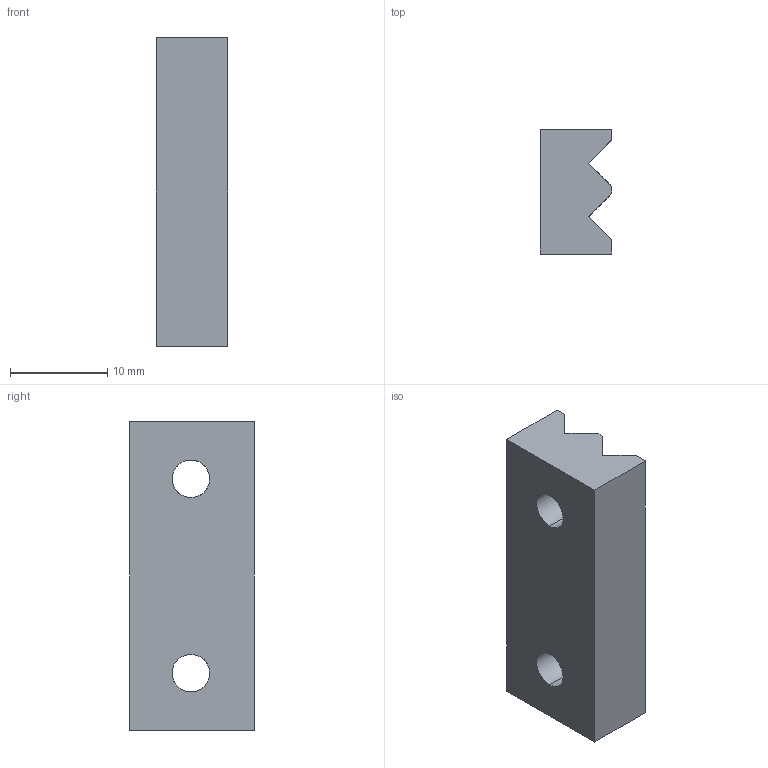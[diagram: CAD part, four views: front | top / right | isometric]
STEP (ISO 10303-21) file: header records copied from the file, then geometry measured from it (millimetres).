
FILE_DESCRIPTION (( 'STEP AP214' ), '1' );
FILE_NAME ('ForeGrip-Retainer.STEP', '2015-01-24T03:30:35', ( 'WarFairy' ), ( '' ), 'SwSTEP 2.0', 'SolidWorks 2013', '' );
FILE_SCHEMA (( 'AUTOMOTIVE_DESIGN' ));
Length unit declared in the file: inch
Products named in the file (1): ForeGrip-Retainer
Bounding box: 7.4 x 12.83 x 31.75 mm (x, y, z)
Volume: 2488.5 mm3; surface area: 1681.1 mm2
Topology: 1 solids, 1 shells, 18 faces, 54 edges, 36 vertices
Faces by surface type: plane 14, cylinder 4
Entity records: 710 total; most frequent: CARTESIAN_POINT 121, ORIENTED_EDGE 108, DIRECTION 100, EDGE_CURVE 54, VECTOR 38, LINE 38, VERTEX_POINT 36, AXIS2_PLACEMENT_3D 31
